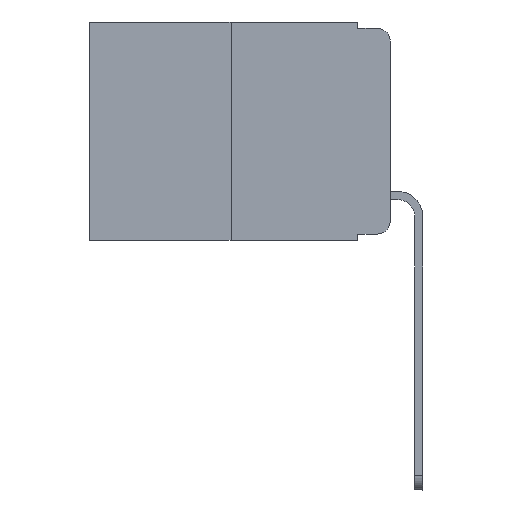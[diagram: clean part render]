
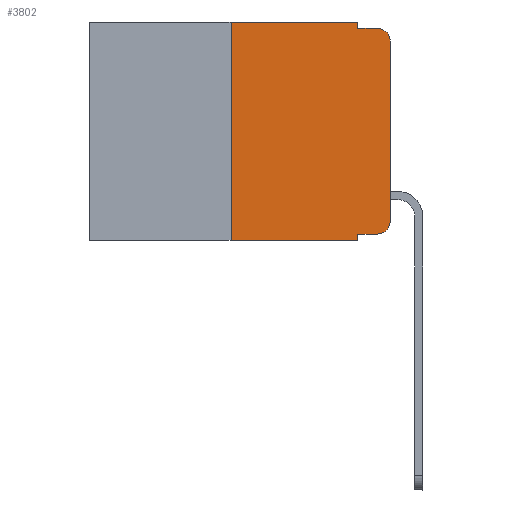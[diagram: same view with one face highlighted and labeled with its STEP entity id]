
A CAD part, left-side view. The second image highlights one B-rep face of the part: STEP entity #3802.
In plain terms, the highlighted planar face has unit normal (-1, 0, 0).
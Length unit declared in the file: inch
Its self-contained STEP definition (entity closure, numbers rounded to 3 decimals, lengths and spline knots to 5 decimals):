
#167 = CARTESIAN_POINT ( 'NONE',  ( 0., 0.051, -0.333 ) ) ;
#267 = EDGE_CURVE ( 'NONE', #15890, #15303, #8088, .T. ) ;
#480 = VECTOR ( 'NONE', #5512, 39.37008 ) ;
#489 = CARTESIAN_POINT ( 'NONE',  ( 0., 0.473, -0.343 ) ) ;
#787 = VERTEX_POINT ( 'NONE', #6556 ) ;
#1468 = LINE ( 'NONE', #4227, #13777 ) ;
#1665 = EDGE_CURVE ( 'NONE', #12010, #3517, #1822, .T. ) ;
#1683 = DIRECTION ( 'NONE',  ( 0., 0., -1. ) ) ;
#1740 = DIRECTION ( 'NONE',  ( 0., 0., -1. ) ) ;
#1822 = LINE ( 'NONE', #9402, #11929 ) ;
#2127 = ORIENTED_EDGE ( 'NONE', *, *, #267, .T. ) ;
#2227 = ORIENTED_EDGE ( 'NONE', *, *, #14129, .F. ) ;
#2646 = LINE ( 'NONE', #7663, #6930 ) ;
#2798 = DIRECTION ( 'NONE',  ( -1., 0., 0. ) ) ;
#2827 = CARTESIAN_POINT ( 'NONE',  ( 0., 0.02, -0.333 ) ) ;
#2927 = VECTOR ( 'NONE', #7005, 39.37008 ) ;
#3073 = ORIENTED_EDGE ( 'NONE', *, *, #11851, .F. ) ;
#3144 = VERTEX_POINT ( 'NONE', #9142 ) ;
#3517 = VERTEX_POINT ( 'NONE', #10185 ) ;
#3802 = ADVANCED_FACE ( 'NONE', ( #14904 ), #14817, .F. ) ;
#3843 = DIRECTION ( 'NONE',  ( 0., 0., 1. ) ) ;
#4227 = CARTESIAN_POINT ( 'NONE',  ( 0., 0., 0. ) ) ;
#4424 = ORIENTED_EDGE ( 'NONE', *, *, #1665, .F. ) ;
#4879 = DIRECTION ( 'NONE',  ( 1., 0., 0. ) ) ;
#5487 = VERTEX_POINT ( 'NONE', #9992 ) ;
#5512 = DIRECTION ( 'NONE',  ( 0., -1., 0. ) ) ;
#6410 = EDGE_CURVE ( 'NONE', #12010, #7323, #12514, .T. ) ;
#6483 = ORIENTED_EDGE ( 'NONE', *, *, #8628, .F. ) ;
#6556 = CARTESIAN_POINT ( 'NONE',  ( 0., 0.051, 0. ) ) ;
#6782 = EDGE_CURVE ( 'NONE', #7323, #3144, #14969, .T. ) ;
#6930 = VECTOR ( 'NONE', #16254, 39.37008 ) ;
#7005 = DIRECTION ( 'NONE',  ( 0., -1., 0. ) ) ;
#7112 = DIRECTION ( 'NONE',  ( -1., 0., 0. ) ) ;
#7220 = CARTESIAN_POINT ( 'NONE',  ( 0., 0.051, -0.333 ) ) ;
#7323 = VERTEX_POINT ( 'NONE', #2827 ) ;
#7367 = DIRECTION ( 'NONE',  ( 0., 0., -1. ) ) ;
#7663 = CARTESIAN_POINT ( 'NONE',  ( 0., 0.473, 0. ) ) ;
#7988 = EDGE_CURVE ( 'NONE', #14156, #3517, #14617, .T. ) ;
#8088 = CIRCLE ( 'NONE', #12307, 0.02 ) ;
#8245 = CARTESIAN_POINT ( 'NONE',  ( 0., 0., -0.03 ) ) ;
#8624 = CARTESIAN_POINT ( 'NONE',  ( 0., 0.02, -0.313 ) ) ;
#8628 = EDGE_CURVE ( 'NONE', #787, #5487, #10493, .T. ) ;
#8892 = AXIS2_PLACEMENT_3D ( 'NONE', #8624, #7112, #12410 ) ;
#9139 = ORIENTED_EDGE ( 'NONE', *, *, #7988, .T. ) ;
#9142 = CARTESIAN_POINT ( 'NONE',  ( 0., 0., -0.313 ) ) ;
#9287 = DIRECTION ( 'NONE',  ( 0., 0., 1. ) ) ;
#9402 = CARTESIAN_POINT ( 'NONE',  ( 0., 0.051, 0. ) ) ;
#9410 = VECTOR ( 'NONE', #1683, 39.37008 ) ;
#9743 = CARTESIAN_POINT ( 'NONE',  ( 0., 0.051, -0.01 ) ) ;
#9755 = CARTESIAN_POINT ( 'NONE',  ( 0., 0.473, 0. ) ) ;
#9874 = CARTESIAN_POINT ( 'NONE',  ( 0., 0.25, 0. ) ) ;
#9992 = CARTESIAN_POINT ( 'NONE',  ( 0., 0.051, -0.01 ) ) ;
#10061 = CARTESIAN_POINT ( 'NONE',  ( 0., 0.02, -0.03 ) ) ;
#10115 = CARTESIAN_POINT ( 'NONE',  ( 0., 0.25, 0. ) ) ;
#10171 = ORIENTED_EDGE ( 'NONE', *, *, #6410, .T. ) ;
#10185 = CARTESIAN_POINT ( 'NONE',  ( 0., 0.051, -0.343 ) ) ;
#10493 = LINE ( 'NONE', #11820, #9410 ) ;
#11243 = AXIS2_PLACEMENT_3D ( 'NONE', #9755, #4879, #7367 ) ;
#11357 = EDGE_LOOP ( 'NONE', ( #14151, #2127, #3073, #6483, #12549, #2227, #9139, #4424, #10171, #15783 ) ) ;
#11617 = VECTOR ( 'NONE', #13436, 39.37008 ) ;
#11820 = CARTESIAN_POINT ( 'NONE',  ( 0., 0.051, 0. ) ) ;
#11851 = EDGE_CURVE ( 'NONE', #5487, #15303, #13317, .T. ) ;
#11929 = VECTOR ( 'NONE', #1740, 39.37008 ) ;
#12010 = VERTEX_POINT ( 'NONE', #167 ) ;
#12307 = AXIS2_PLACEMENT_3D ( 'NONE', #10061, #2798, #12710 ) ;
#12410 = DIRECTION ( 'NONE',  ( 0., 0., -1. ) ) ;
#12514 = LINE ( 'NONE', #7220, #11617 ) ;
#12549 = ORIENTED_EDGE ( 'NONE', *, *, #16074, .F. ) ;
#12710 = DIRECTION ( 'NONE',  ( 0., 0., -1. ) ) ;
#12839 = CARTESIAN_POINT ( 'NONE',  ( 0., 0.02, -0.01 ) ) ;
#13050 = EDGE_CURVE ( 'NONE', #3144, #15890, #1468, .T. ) ;
#13317 = LINE ( 'NONE', #9743, #2927 ) ;
#13436 = DIRECTION ( 'NONE',  ( 0., -1., 0. ) ) ;
#13498 = VECTOR ( 'NONE', #3843, 39.37008 ) ;
#13777 = VECTOR ( 'NONE', #9287, 39.37008 ) ;
#13856 = LINE ( 'NONE', #9874, #13498 ) ;
#13938 = CARTESIAN_POINT ( 'NONE',  ( 0., 0.25, -0.343 ) ) ;
#14129 = EDGE_CURVE ( 'NONE', #14156, #15178, #13856, .T. ) ;
#14151 = ORIENTED_EDGE ( 'NONE', *, *, #13050, .T. ) ;
#14156 = VERTEX_POINT ( 'NONE', #13938 ) ;
#14617 = LINE ( 'NONE', #489, #480 ) ;
#14817 = PLANE ( 'NONE',  #11243 ) ;
#14904 = FACE_OUTER_BOUND ( 'NONE', #11357, .T. ) ;
#14969 = CIRCLE ( 'NONE', #8892, 0.02 ) ;
#15178 = VERTEX_POINT ( 'NONE', #10115 ) ;
#15303 = VERTEX_POINT ( 'NONE', #12839 ) ;
#15783 = ORIENTED_EDGE ( 'NONE', *, *, #6782, .T. ) ;
#15890 = VERTEX_POINT ( 'NONE', #8245 ) ;
#16074 = EDGE_CURVE ( 'NONE', #15178, #787, #2646, .T. ) ;
#16254 = DIRECTION ( 'NONE',  ( 0., -1., 0. ) ) ;
